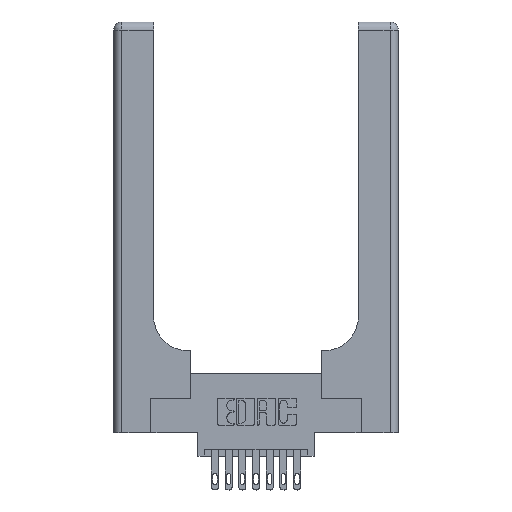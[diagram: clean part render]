
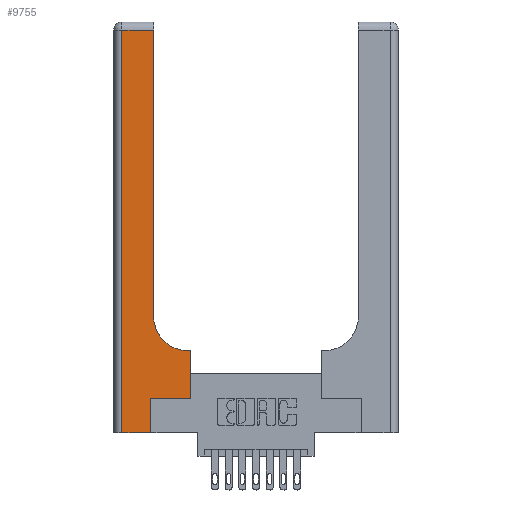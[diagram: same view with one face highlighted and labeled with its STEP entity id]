
A CAD part, top view. The second image highlights one B-rep face of the part: STEP entity #9755.
In plain terms, the highlighted planar face has unit normal (0, 0, 1).
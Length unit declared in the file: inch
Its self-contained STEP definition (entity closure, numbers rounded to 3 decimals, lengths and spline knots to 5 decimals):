
#517 = EDGE_CURVE ( 'NONE', #13466, #8451, #3304, .T. ) ;
#874 = ORIENTED_EDGE ( 'NONE', *, *, #3657, .T. ) ;
#889 = CARTESIAN_POINT ( 'NONE',  ( 0.06, 0., 0.37 ) ) ;
#1536 = VECTOR ( 'NONE', #14024, 39.37008 ) ;
#1907 = FACE_OUTER_BOUND ( 'NONE', #15218, .T. ) ;
#1917 = DIRECTION ( 'NONE',  ( 1., 0., 0. ) ) ;
#1962 = DIRECTION ( 'NONE',  ( 1., 0., 0. ) ) ;
#2192 = VERTEX_POINT ( 'NONE', #7086 ) ;
#2322 = EDGE_CURVE ( 'NONE', #10840, #11855, #3613, .T. ) ;
#2364 = LINE ( 'NONE', #4962, #5149 ) ;
#2767 = CARTESIAN_POINT ( 'NONE',  ( 0.06, 3., 0.37 ) ) ;
#2840 = VECTOR ( 'NONE', #10590, 39.37008 ) ;
#2891 = CIRCLE ( 'NONE', #5939, 0.25 ) ;
#3304 = LINE ( 'NONE', #14426, #9611 ) ;
#3574 = CARTESIAN_POINT ( 'NONE',  ( 0.5585, 0.25, 0.37 ) ) ;
#3613 = LINE ( 'NONE', #11699, #13687 ) ;
#3657 = EDGE_CURVE ( 'NONE', #8451, #12017, #5819, .T. ) ;
#3790 = DIRECTION ( 'NONE',  ( -1., 0., 0. ) ) ;
#3832 = EDGE_CURVE ( 'NONE', #5762, #13466, #4691, .T. ) ;
#4189 = DIRECTION ( 'NONE',  ( 0., 0., -1. ) ) ;
#4222 = ORIENTED_EDGE ( 'NONE', *, *, #3832, .T. ) ;
#4539 = EDGE_CURVE ( 'NONE', #2192, #5762, #12927, .T. ) ;
#4691 = LINE ( 'NONE', #2767, #1536 ) ;
#4962 = CARTESIAN_POINT ( 'NONE',  ( 0.2915, 0.6, 0.37 ) ) ;
#5149 = VECTOR ( 'NONE', #12239, 39.37008 ) ;
#5220 = VECTOR ( 'NONE', #9175, 39.37008 ) ;
#5359 = ORIENTED_EDGE ( 'NONE', *, *, #2322, .T. ) ;
#5489 = CARTESIAN_POINT ( 'NONE',  ( 0.5415, 0.85, 0.37 ) ) ;
#5762 = VERTEX_POINT ( 'NONE', #6656 ) ;
#5819 = LINE ( 'NONE', #6419, #13107 ) ;
#5865 = ORIENTED_EDGE ( 'NONE', *, *, #13440, .T. ) ;
#5939 = AXIS2_PLACEMENT_3D ( 'NONE', #5489, #4189, #1962 ) ;
#6282 = CARTESIAN_POINT ( 'NONE',  ( 0., 3., 0.37 ) ) ;
#6334 = DIRECTION ( 'NONE',  ( 0., 0., -1. ) ) ;
#6419 = CARTESIAN_POINT ( 'NONE',  ( 0.269, 0., 0.37 ) ) ;
#6656 = CARTESIAN_POINT ( 'NONE',  ( 0.06, 2.94, 0.37 ) ) ;
#6892 = CARTESIAN_POINT ( 'NONE',  ( 0., 2.94, 0.37 ) ) ;
#6901 = CARTESIAN_POINT ( 'NONE',  ( 0.2915, 0.85, 0.37 ) ) ;
#6928 = EDGE_CURVE ( 'NONE', #11855, #10806, #2364, .T. ) ;
#7086 = CARTESIAN_POINT ( 'NONE',  ( 0.2915, 2.94, 0.37 ) ) ;
#7348 = DIRECTION ( 'NONE',  ( 0., 1., 0. ) ) ;
#7730 = CARTESIAN_POINT ( 'NONE',  ( 0.5585, 0.6, 0.37 ) ) ;
#7768 = ORIENTED_EDGE ( 'NONE', *, *, #9505, .T. ) ;
#8429 = DIRECTION ( 'NONE',  ( 1., 0., 0. ) ) ;
#8448 = VERTEX_POINT ( 'NONE', #6901 ) ;
#8451 = VERTEX_POINT ( 'NONE', #14105 ) ;
#9084 = CARTESIAN_POINT ( 'NONE',  ( 0.269, 0.25, 0.37 ) ) ;
#9175 = DIRECTION ( 'NONE',  ( -1., 0., 0. ) ) ;
#9372 = CARTESIAN_POINT ( 'NONE',  ( 0.2915, 3., 0.37 ) ) ;
#9505 = EDGE_CURVE ( 'NONE', #8448, #2192, #12193, .T. ) ;
#9587 = CARTESIAN_POINT ( 'NONE',  ( 0.5415, 0.6, 0.37 ) ) ;
#9611 = VECTOR ( 'NONE', #8429, 39.37008 ) ;
#9755 = ADVANCED_FACE ( 'NONE', ( #1907 ), #10931, .F. ) ;
#10193 = AXIS2_PLACEMENT_3D ( 'NONE', #6282, #6334, #3790 ) ;
#10590 = DIRECTION ( 'NONE',  ( 0., 1., 0. ) ) ;
#10806 = VERTEX_POINT ( 'NONE', #9587 ) ;
#10840 = VERTEX_POINT ( 'NONE', #3574 ) ;
#10931 = PLANE ( 'NONE',  #10193 ) ;
#11243 = DIRECTION ( 'NONE',  ( 0., 1., 0. ) ) ;
#11256 = ORIENTED_EDGE ( 'NONE', *, *, #517, .T. ) ;
#11312 = CARTESIAN_POINT ( 'NONE',  ( 0.269, 0.25, 0.37 ) ) ;
#11692 = VECTOR ( 'NONE', #1917, 39.37008 ) ;
#11699 = CARTESIAN_POINT ( 'NONE',  ( 0.5585, 0.25, 0.37 ) ) ;
#11855 = VERTEX_POINT ( 'NONE', #7730 ) ;
#11924 = EDGE_CURVE ( 'NONE', #12017, #10840, #14861, .T. ) ;
#12017 = VERTEX_POINT ( 'NONE', #9084 ) ;
#12193 = LINE ( 'NONE', #9372, #2840 ) ;
#12239 = DIRECTION ( 'NONE',  ( -1., 0., 0. ) ) ;
#12549 = ORIENTED_EDGE ( 'NONE', *, *, #4539, .T. ) ;
#12927 = LINE ( 'NONE', #6892, #5220 ) ;
#12983 = ORIENTED_EDGE ( 'NONE', *, *, #11924, .T. ) ;
#13107 = VECTOR ( 'NONE', #7348, 39.37008 ) ;
#13440 = EDGE_CURVE ( 'NONE', #10806, #8448, #2891, .T. ) ;
#13466 = VERTEX_POINT ( 'NONE', #889 ) ;
#13687 = VECTOR ( 'NONE', #11243, 39.37008 ) ;
#14024 = DIRECTION ( 'NONE',  ( 0., -1., 0. ) ) ;
#14105 = CARTESIAN_POINT ( 'NONE',  ( 0.269, 0., 0.37 ) ) ;
#14426 = CARTESIAN_POINT ( 'NONE',  ( 0., 0., 0.37 ) ) ;
#14861 = LINE ( 'NONE', #11312, #11692 ) ;
#15218 = EDGE_LOOP ( 'NONE', ( #7768, #12549, #4222, #11256, #874, #12983, #5359, #15275, #5865 ) ) ;
#15275 = ORIENTED_EDGE ( 'NONE', *, *, #6928, .T. ) ;
